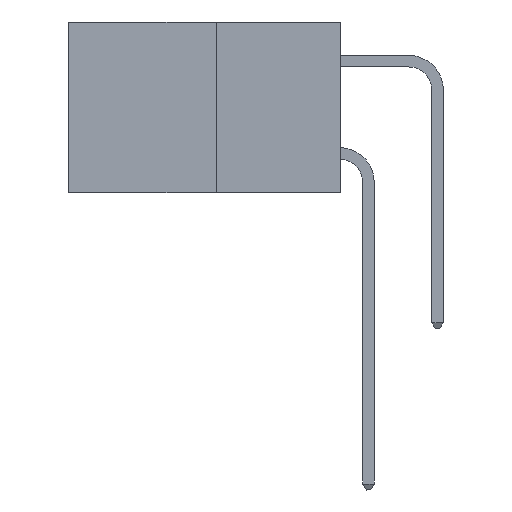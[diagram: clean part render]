
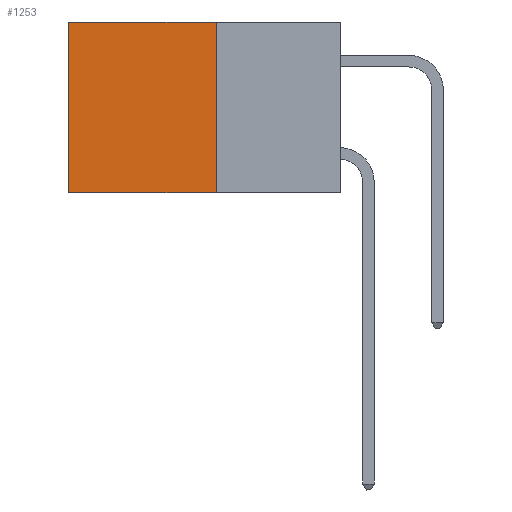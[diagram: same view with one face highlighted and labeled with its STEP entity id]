
A CAD part, left-side view. The second image highlights one B-rep face of the part: STEP entity #1253.
In plain terms, the highlighted planar face has unit normal (-1, 0, 0).
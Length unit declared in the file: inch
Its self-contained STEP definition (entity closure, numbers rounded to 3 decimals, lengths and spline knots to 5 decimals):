
#238 = CARTESIAN_POINT ( 'NONE',  ( 0.277, 0.27, -0.37 ) ) ;
#812 = VERTEX_POINT ( 'NONE', #6681 ) ;
#1253 = ADVANCED_FACE ( 'NONE', ( #11144 ), #19730, .F. ) ;
#1536 = CARTESIAN_POINT ( 'NONE',  ( 0.277, 0.27, -0.37 ) ) ;
#1953 = VERTEX_POINT ( 'NONE', #238 ) ;
#2629 = ORIENTED_EDGE ( 'NONE', *, *, #5779, .T. ) ;
#3486 = VECTOR ( 'NONE', #17345, 39.37008 ) ;
#3835 = VERTEX_POINT ( 'NONE', #8791 ) ;
#5452 = EDGE_CURVE ( 'NONE', #3835, #1953, #11671, .T. ) ;
#5779 = EDGE_CURVE ( 'NONE', #812, #16032, #6383, .T. ) ;
#6383 = LINE ( 'NONE', #12031, #14598 ) ;
#6566 = EDGE_CURVE ( 'NONE', #1953, #16032, #11856, .T. ) ;
#6681 = CARTESIAN_POINT ( 'NONE',  ( 0.277, 0.59, 0. ) ) ;
#7264 = ORIENTED_EDGE ( 'NONE', *, *, #6566, .F. ) ;
#7668 = VECTOR ( 'NONE', #13035, 39.37008 ) ;
#7794 = ORIENTED_EDGE ( 'NONE', *, *, #11674, .T. ) ;
#7797 = VECTOR ( 'NONE', #16132, 39.37008 ) ;
#8791 = CARTESIAN_POINT ( 'NONE',  ( 0.277, 0.27, 0. ) ) ;
#11144 = FACE_OUTER_BOUND ( 'NONE', #13548, .T. ) ;
#11671 = LINE ( 'NONE', #16483, #3486 ) ;
#11674 = EDGE_CURVE ( 'NONE', #3835, #812, #19456, .T. ) ;
#11856 = LINE ( 'NONE', #19167, #7797 ) ;
#11918 = DIRECTION ( 'NONE',  ( 0., 0., -1. ) ) ;
#12031 = CARTESIAN_POINT ( 'NONE',  ( 0.277, 0.59, -0.37 ) ) ;
#13035 = DIRECTION ( 'NONE',  ( 0., 1., 0. ) ) ;
#13548 = EDGE_LOOP ( 'NONE', ( #2629, #7264, #16549, #7794 ) ) ;
#14108 = CARTESIAN_POINT ( 'NONE',  ( 0.277, 0.59, -0.37 ) ) ;
#14598 = VECTOR ( 'NONE', #11918, 39.37008 ) ;
#16032 = VERTEX_POINT ( 'NONE', #14108 ) ;
#16132 = DIRECTION ( 'NONE',  ( 0., 1., 0. ) ) ;
#16483 = CARTESIAN_POINT ( 'NONE',  ( 0.277, 0.27, -0.37 ) ) ;
#16549 = ORIENTED_EDGE ( 'NONE', *, *, #5452, .F. ) ;
#16715 = AXIS2_PLACEMENT_3D ( 'NONE', #1536, #19522, #19508 ) ;
#17345 = DIRECTION ( 'NONE',  ( 0., 0., -1. ) ) ;
#17735 = CARTESIAN_POINT ( 'NONE',  ( 0.277, 0.27, 0. ) ) ;
#19167 = CARTESIAN_POINT ( 'NONE',  ( 0.277, 0.27, -0.37 ) ) ;
#19456 = LINE ( 'NONE', #17735, #7668 ) ;
#19508 = DIRECTION ( 'NONE',  ( 0., 0., -1. ) ) ;
#19522 = DIRECTION ( 'NONE',  ( 1., 0., 0. ) ) ;
#19730 = PLANE ( 'NONE',  #16715 ) ;
